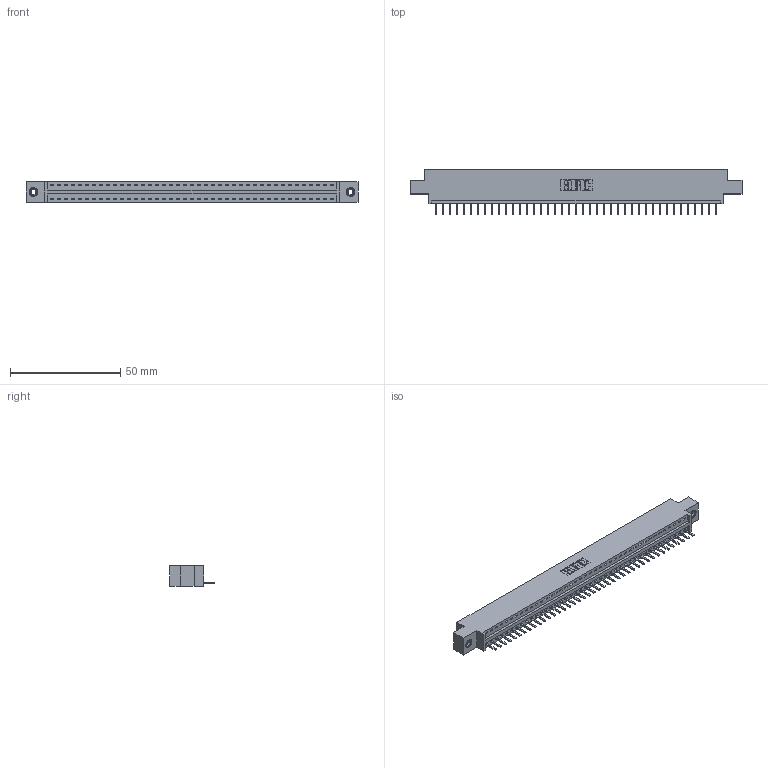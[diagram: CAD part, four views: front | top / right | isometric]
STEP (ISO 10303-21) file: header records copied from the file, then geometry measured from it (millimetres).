
FILE_DESCRIPTION (( 'STEP AP203' ), '1' );
FILE_NAME ('396-041-520-608.STEP', '2018-09-06T22:16:26', ( '' ), ( '' ), 'SwSTEP 2.0', 'SolidWorks 2016', '' );
FILE_SCHEMA (( 'CONFIG_CONTROL_DESIGN' ));
Length unit declared in the file: inch
Products named in the file (4): 346 Part_0.170 Offset - 0.156 Dia-TI; 345-292-001_345-293-120; 345-250-001_345-250-003-102; 396-041-520-608
Assembly tree (44 placements, depth 2):
  396-041-520-608
    346 Part_0.170 Offset - 0.156 Dia-TI
    345-292-001_345-293-120  x41
    345-250-001_345-250-003-102  x2
Bounding box: 150.75 x 20.02 x 9.4 mm (x, y, z)
Volume: 14144.1 mm3; surface area: 17455.9 mm2
Topology: 44 solids, 44 shells, 2728 faces, 8021 edges, 5230 vertices
Faces by surface type: plane 1834, cylinder 878, cone 12, torus 4
Entity records: 27012 total; most frequent: CARTESIAN_POINT 4626, ORIENTED_EDGE 4582, DIRECTION 4095, EDGE_CURVE 2291, LINE 1971, VECTOR 1971, VERTEX_POINT 1520, AXIS2_PLACEMENT_3D 1062
